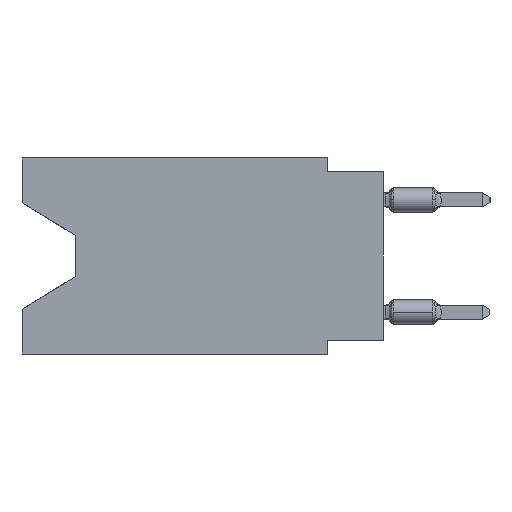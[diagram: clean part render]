
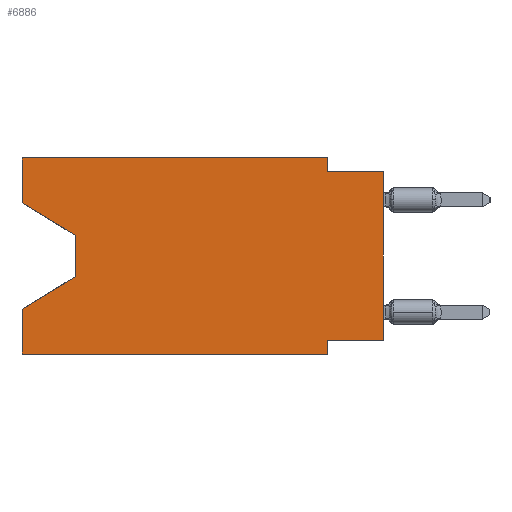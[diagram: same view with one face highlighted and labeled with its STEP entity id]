
A CAD part, left-side view. The second image highlights one B-rep face of the part: STEP entity #6886.
In plain terms, the highlighted planar face has unit normal (-1, 0, 0).
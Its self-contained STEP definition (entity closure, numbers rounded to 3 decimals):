
#280 = CARTESIAN_POINT ( 'NONE',  ( 0., 13.97, -3.505 ) ) ;
#360 = VERTEX_POINT ( 'NONE', #981 ) ;
#505 = EDGE_CURVE ( 'NONE', #10341, #22041, #23897, .T. ) ;
#661 = ORIENTED_EDGE ( 'NONE', *, *, #24576, .T. ) ;
#851 = CARTESIAN_POINT ( 'NONE',  ( 0., 16.383, 0. ) ) ;
#981 = CARTESIAN_POINT ( 'NONE',  ( 0., 2.54, -8.89 ) ) ;
#1131 = VECTOR ( 'NONE', #23060, 1000. ) ;
#1178 = CARTESIAN_POINT ( 'NONE',  ( 0., 0., -8.255 ) ) ;
#1469 = EDGE_CURVE ( 'NONE', #17563, #10341, #14218, .T. ) ;
#2795 = CARTESIAN_POINT ( 'NONE',  ( 0., 16.383, 0. ) ) ;
#2888 = CARTESIAN_POINT ( 'NONE',  ( 0., 0., -0.635 ) ) ;
#3588 = VERTEX_POINT ( 'NONE', #25785 ) ;
#3813 = ORIENTED_EDGE ( 'NONE', *, *, #7348, .F. ) ;
#3944 = VERTEX_POINT ( 'NONE', #11826 ) ;
#3977 = LINE ( 'NONE', #851, #15536 ) ;
#4043 = LINE ( 'NONE', #21785, #13920 ) ;
#4547 = VERTEX_POINT ( 'NONE', #8600 ) ;
#5171 = ORIENTED_EDGE ( 'NONE', *, *, #20019, .F. ) ;
#5397 = EDGE_CURVE ( 'NONE', #3588, #360, #10893, .T. ) ;
#5509 = CARTESIAN_POINT ( 'NONE',  ( 0., 0., -0.635 ) ) ;
#6518 = DIRECTION ( 'NONE',  ( 0., 0., 1. ) ) ;
#6886 = ADVANCED_FACE ( 'NONE', ( #7726 ), #26134, .F. ) ;
#7009 = VECTOR ( 'NONE', #6518, 1000. ) ;
#7301 = LINE ( 'NONE', #15510, #20855 ) ;
#7348 = EDGE_CURVE ( 'NONE', #17956, #3944, #15868, .T. ) ;
#7416 = ORIENTED_EDGE ( 'NONE', *, *, #10655, .F. ) ;
#7726 = FACE_OUTER_BOUND ( 'NONE', #10959, .T. ) ;
#8336 = EDGE_CURVE ( 'NONE', #14602, #360, #7301, .T. ) ;
#8600 = CARTESIAN_POINT ( 'NONE',  ( 0., 2.54, -0.635 ) ) ;
#8618 = ORIENTED_EDGE ( 'NONE', *, *, #22696, .F. ) ;
#8651 = ORIENTED_EDGE ( 'NONE', *, *, #505, .T. ) ;
#8652 = ORIENTED_EDGE ( 'NONE', *, *, #15266, .F. ) ;
#9404 = LINE ( 'NONE', #1178, #21252 ) ;
#10341 = VERTEX_POINT ( 'NONE', #25448 ) ;
#10655 = EDGE_CURVE ( 'NONE', #19009, #14602, #9404, .T. ) ;
#10893 = LINE ( 'NONE', #12490, #1131 ) ;
#10959 = EDGE_LOOP ( 'NONE', ( #661, #14860, #8651, #8652, #23971, #21453, #7416, #16669, #5171, #25583, #3813, #8618 ) ) ;
#11484 = CARTESIAN_POINT ( 'NONE',  ( 0., 16.383, -2.038 ) ) ;
#11639 = DIRECTION ( 'NONE',  ( 0., 0., 1. ) ) ;
#11826 = CARTESIAN_POINT ( 'NONE',  ( 0., 2.54, 0. ) ) ;
#11836 = CARTESIAN_POINT ( 'NONE',  ( 0., 16.383, -2.038 ) ) ;
#12021 = VECTOR ( 'NONE', #12043, 1000. ) ;
#12043 = DIRECTION ( 'NONE',  ( 0., -1., 0. ) ) ;
#12490 = CARTESIAN_POINT ( 'NONE',  ( 0., 16.383, -8.89 ) ) ;
#12681 = EDGE_CURVE ( 'NONE', #19009, #13764, #15460, .T. ) ;
#12993 = DIRECTION ( 'NONE',  ( 0., 1., 0. ) ) ;
#13764 = VERTEX_POINT ( 'NONE', #2888 ) ;
#13920 = VECTOR ( 'NONE', #20312, 1000. ) ;
#13945 = DIRECTION ( 'NONE',  ( 0., -0.855, -0.519 ) ) ;
#14218 = LINE ( 'NONE', #280, #24258 ) ;
#14602 = VERTEX_POINT ( 'NONE', #15133 ) ;
#14860 = ORIENTED_EDGE ( 'NONE', *, *, #1469, .T. ) ;
#15133 = CARTESIAN_POINT ( 'NONE',  ( 0., 2.54, -8.255 ) ) ;
#15266 = EDGE_CURVE ( 'NONE', #3588, #22041, #3977, .T. ) ;
#15460 = LINE ( 'NONE', #25657, #26118 ) ;
#15510 = CARTESIAN_POINT ( 'NONE',  ( 0., 2.54, -8.89 ) ) ;
#15536 = VECTOR ( 'NONE', #16276, 1000. ) ;
#15595 = VECTOR ( 'NONE', #21399, 1000. ) ;
#15821 = CARTESIAN_POINT ( 'NONE',  ( 0., 13.97, -5.385 ) ) ;
#15868 = LINE ( 'NONE', #18132, #12021 ) ;
#16019 = VECTOR ( 'NONE', #19922, 1000. ) ;
#16276 = DIRECTION ( 'NONE',  ( 0., 0., 1. ) ) ;
#16669 = ORIENTED_EDGE ( 'NONE', *, *, #12681, .T. ) ;
#16688 = AXIS2_PLACEMENT_3D ( 'NONE', #25870, #21770, #18067 ) ;
#17563 = VERTEX_POINT ( 'NONE', #23090 ) ;
#17956 = VERTEX_POINT ( 'NONE', #2795 ) ;
#18067 = DIRECTION ( 'NONE',  ( 0., 0., -1. ) ) ;
#18132 = CARTESIAN_POINT ( 'NONE',  ( 0., 16.383, 0. ) ) ;
#19009 = VERTEX_POINT ( 'NONE', #22008 ) ;
#19068 = VECTOR ( 'NONE', #13945, 1000. ) ;
#19922 = DIRECTION ( 'NONE',  ( 0., 0.855, -0.519 ) ) ;
#19962 = VERTEX_POINT ( 'NONE', #11484 ) ;
#20019 = EDGE_CURVE ( 'NONE', #4547, #13764, #23644, .T. ) ;
#20037 = EDGE_CURVE ( 'NONE', #3944, #4547, #4043, .T. ) ;
#20312 = DIRECTION ( 'NONE',  ( 0., 0., -1. ) ) ;
#20855 = VECTOR ( 'NONE', #23591, 1000. ) ;
#21252 = VECTOR ( 'NONE', #12993, 1000. ) ;
#21399 = DIRECTION ( 'NONE',  ( 0., -1., 0. ) ) ;
#21453 = ORIENTED_EDGE ( 'NONE', *, *, #8336, .F. ) ;
#21770 = DIRECTION ( 'NONE',  ( 1., 0., 0. ) ) ;
#21785 = CARTESIAN_POINT ( 'NONE',  ( 0., 2.54, 0. ) ) ;
#22008 = CARTESIAN_POINT ( 'NONE',  ( 0., 0., -8.255 ) ) ;
#22041 = VERTEX_POINT ( 'NONE', #23780 ) ;
#22696 = EDGE_CURVE ( 'NONE', #19962, #17956, #24400, .T. ) ;
#23060 = DIRECTION ( 'NONE',  ( 0., -1., 0. ) ) ;
#23090 = CARTESIAN_POINT ( 'NONE',  ( 0., 13.97, -3.505 ) ) ;
#23591 = DIRECTION ( 'NONE',  ( 0., 0., -1. ) ) ;
#23644 = LINE ( 'NONE', #5509, #15595 ) ;
#23780 = CARTESIAN_POINT ( 'NONE',  ( 0., 16.383, -6.852 ) ) ;
#23868 = LINE ( 'NONE', #11836, #19068 ) ;
#23897 = LINE ( 'NONE', #15821, #16019 ) ;
#23971 = ORIENTED_EDGE ( 'NONE', *, *, #5397, .T. ) ;
#24258 = VECTOR ( 'NONE', #24790, 1000. ) ;
#24400 = LINE ( 'NONE', #24655, #7009 ) ;
#24576 = EDGE_CURVE ( 'NONE', #19962, #17563, #23868, .T. ) ;
#24655 = CARTESIAN_POINT ( 'NONE',  ( 0., 16.383, 0. ) ) ;
#24790 = DIRECTION ( 'NONE',  ( 0., 0., -1. ) ) ;
#25448 = CARTESIAN_POINT ( 'NONE',  ( 0., 13.97, -5.385 ) ) ;
#25583 = ORIENTED_EDGE ( 'NONE', *, *, #20037, .F. ) ;
#25657 = CARTESIAN_POINT ( 'NONE',  ( 0., 0., 0. ) ) ;
#25785 = CARTESIAN_POINT ( 'NONE',  ( 0., 16.383, -8.89 ) ) ;
#25870 = CARTESIAN_POINT ( 'NONE',  ( 0., 16.383, 0. ) ) ;
#26118 = VECTOR ( 'NONE', #11639, 1000. ) ;
#26134 = PLANE ( 'NONE',  #16688 ) ;
